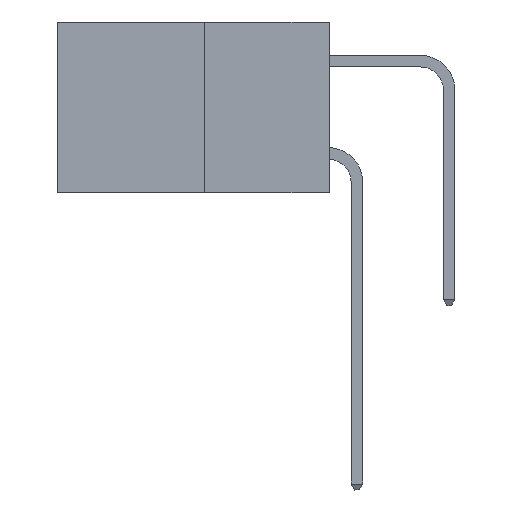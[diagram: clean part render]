
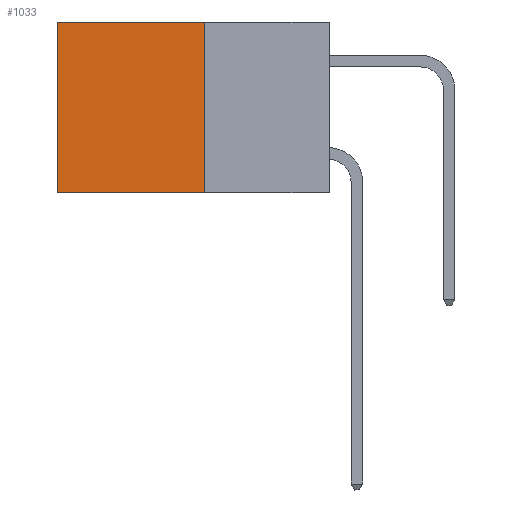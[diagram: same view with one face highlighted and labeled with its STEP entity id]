
A CAD part, left-side view. The second image highlights one B-rep face of the part: STEP entity #1033.
In plain terms, the highlighted planar face has unit normal (-1, 0, 0).
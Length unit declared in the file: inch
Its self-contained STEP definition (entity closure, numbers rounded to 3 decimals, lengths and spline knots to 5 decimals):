
#2 = DIRECTION ( 'NONE',  ( 0., 0., -1. ) ) ;
#763 = EDGE_CURVE ( 'NONE', #12876, #3094, #15075, .T. ) ;
#872 = EDGE_CURVE ( 'NONE', #15314, #3094, #13265, .T. ) ;
#1033 = ADVANCED_FACE ( 'NONE', ( #3455 ), #18185, .F. ) ;
#1851 = EDGE_CURVE ( 'NONE', #3794, #15314, #4595, .T. ) ;
#2015 = EDGE_LOOP ( 'NONE', ( #12466, #15287, #3960, #16670 ) ) ;
#2295 = CARTESIAN_POINT ( 'NONE',  ( 0.277, 0.59, -0.37 ) ) ;
#3094 = VERTEX_POINT ( 'NONE', #16324 ) ;
#3101 = CARTESIAN_POINT ( 'NONE',  ( 0.277, 0.27, 0. ) ) ;
#3455 = FACE_OUTER_BOUND ( 'NONE', #2015, .T. ) ;
#3794 = VERTEX_POINT ( 'NONE', #17542 ) ;
#3960 = ORIENTED_EDGE ( 'NONE', *, *, #14959, .F. ) ;
#4536 = VECTOR ( 'NONE', #10312, 39.37008 ) ;
#4595 = LINE ( 'NONE', #3101, #15081 ) ;
#5371 = CARTESIAN_POINT ( 'NONE',  ( 0.277, 0.59, 0. ) ) ;
#7149 = DIRECTION ( 'NONE',  ( 1., 0., 0. ) ) ;
#7736 = DIRECTION ( 'NONE',  ( 0., 1., 0. ) ) ;
#8382 = LINE ( 'NONE', #14579, #4536 ) ;
#10024 = CARTESIAN_POINT ( 'NONE',  ( 0.277, 0.27, -0.37 ) ) ;
#10233 = AXIS2_PLACEMENT_3D ( 'NONE', #12335, #7149, #2 ) ;
#10312 = DIRECTION ( 'NONE',  ( 0., 0., -1. ) ) ;
#12335 = CARTESIAN_POINT ( 'NONE',  ( 0.277, 0.27, -0.37 ) ) ;
#12466 = ORIENTED_EDGE ( 'NONE', *, *, #872, .T. ) ;
#12876 = VERTEX_POINT ( 'NONE', #10024 ) ;
#13265 = LINE ( 'NONE', #2295, #16160 ) ;
#13988 = CARTESIAN_POINT ( 'NONE',  ( 0.277, 0.27, -0.37 ) ) ;
#14020 = DIRECTION ( 'NONE',  ( 0., 0., -1. ) ) ;
#14254 = DIRECTION ( 'NONE',  ( 0., 1., 0. ) ) ;
#14579 = CARTESIAN_POINT ( 'NONE',  ( 0.277, 0.27, -0.37 ) ) ;
#14959 = EDGE_CURVE ( 'NONE', #3794, #12876, #8382, .T. ) ;
#15075 = LINE ( 'NONE', #13988, #18365 ) ;
#15081 = VECTOR ( 'NONE', #14254, 39.37008 ) ;
#15287 = ORIENTED_EDGE ( 'NONE', *, *, #763, .F. ) ;
#15314 = VERTEX_POINT ( 'NONE', #5371 ) ;
#16160 = VECTOR ( 'NONE', #14020, 39.37008 ) ;
#16324 = CARTESIAN_POINT ( 'NONE',  ( 0.277, 0.59, -0.37 ) ) ;
#16670 = ORIENTED_EDGE ( 'NONE', *, *, #1851, .T. ) ;
#17542 = CARTESIAN_POINT ( 'NONE',  ( 0.277, 0.27, 0. ) ) ;
#18185 = PLANE ( 'NONE',  #10233 ) ;
#18365 = VECTOR ( 'NONE', #7736, 39.37008 ) ;
